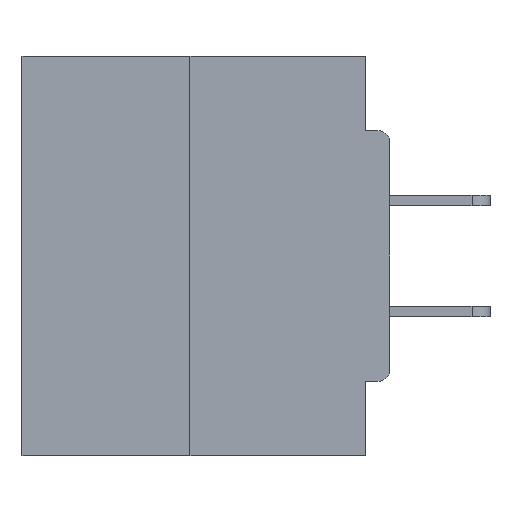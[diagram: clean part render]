
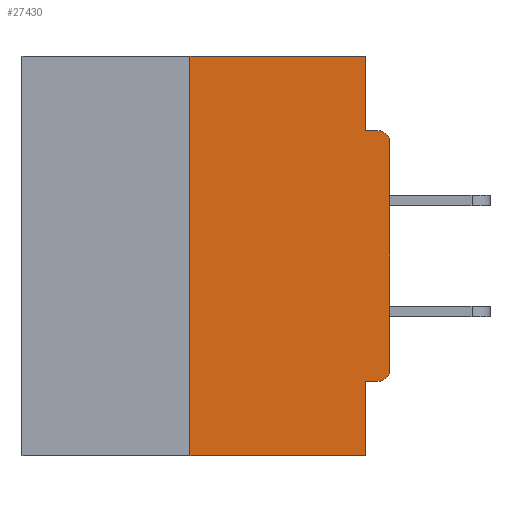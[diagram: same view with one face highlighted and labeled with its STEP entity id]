
A CAD part, left-side view. The second image highlights one B-rep face of the part: STEP entity #27430.
In plain terms, the highlighted planar face has unit normal (-1, 0, 0).
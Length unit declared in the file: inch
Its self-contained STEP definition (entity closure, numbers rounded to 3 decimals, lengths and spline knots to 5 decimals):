
#568 = CARTESIAN_POINT ( 'NONE',  ( 0., 0., -0.4065 ) ) ;
#651 = DIRECTION ( 'NONE',  ( 0., -1., 0. ) ) ;
#1003 = PLANE ( 'NONE',  #7774 ) ;
#1211 = VERTEX_POINT ( 'NONE', #4694 ) ;
#1562 = VERTEX_POINT ( 'NONE', #13886 ) ;
#2189 = CIRCLE ( 'NONE', #25686, 0.015 ) ;
#3286 = VECTOR ( 'NONE', #24534, 39.37008 ) ;
#3760 = VERTEX_POINT ( 'NONE', #14637 ) ;
#3921 = DIRECTION ( 'NONE',  ( 0., 0., -1. ) ) ;
#4142 = EDGE_CURVE ( 'NONE', #23697, #5445, #2189, .T. ) ;
#4460 = CARTESIAN_POINT ( 'NONE',  ( 0., 0.015, -0.1085 ) ) ;
#4552 = LINE ( 'NONE', #12331, #5363 ) ;
#4583 = LINE ( 'NONE', #19253, #12326 ) ;
#4694 = CARTESIAN_POINT ( 'NONE',  ( 0., 0.25, -0.5 ) ) ;
#4850 = DIRECTION ( 'NONE',  ( 0., 0., -1. ) ) ;
#4915 = EDGE_CURVE ( 'NONE', #1211, #28017, #23718, .T. ) ;
#5363 = VECTOR ( 'NONE', #28226, 39.37008 ) ;
#5445 = VERTEX_POINT ( 'NONE', #30517 ) ;
#5545 = EDGE_CURVE ( 'NONE', #1211, #30929, #17136, .T. ) ;
#7144 = LINE ( 'NONE', #28218, #26392 ) ;
#7532 = CIRCLE ( 'NONE', #31305, 0.015 ) ;
#7774 = AXIS2_PLACEMENT_3D ( 'NONE', #29403, #24386, #29758 ) ;
#8301 = VERTEX_POINT ( 'NONE', #27551 ) ;
#8488 = DIRECTION ( 'NONE',  ( 0., 0., -1. ) ) ;
#8930 = CARTESIAN_POINT ( 'NONE',  ( 0., 0.25, 0. ) ) ;
#9136 = CARTESIAN_POINT ( 'NONE',  ( 0., 0.031, -0.5 ) ) ;
#9816 = LINE ( 'NONE', #568, #31940 ) ;
#11010 = DIRECTION ( 'NONE',  ( 0., 1., 0. ) ) ;
#11170 = ORIENTED_EDGE ( 'NONE', *, *, #29361, .T. ) ;
#11292 = EDGE_CURVE ( 'NONE', #30929, #8301, #4552, .T. ) ;
#11531 = ORIENTED_EDGE ( 'NONE', *, *, #11292, .F. ) ;
#11985 = DIRECTION ( 'NONE',  ( -1., 0., 0. ) ) ;
#12326 = VECTOR ( 'NONE', #8488, 39.37008 ) ;
#12327 = VECTOR ( 'NONE', #20142, 39.37008 ) ;
#12331 = CARTESIAN_POINT ( 'NONE',  ( 0., 0.46, 0. ) ) ;
#13746 = CARTESIAN_POINT ( 'NONE',  ( 0., 0.031, -0.0935 ) ) ;
#13886 = CARTESIAN_POINT ( 'NONE',  ( 0., 0.015, -0.4065 ) ) ;
#13926 = CARTESIAN_POINT ( 'NONE',  ( 0., 0., -0.1085 ) ) ;
#13943 = DIRECTION ( 'NONE',  ( -1., 0., 0. ) ) ;
#14561 = ORIENTED_EDGE ( 'NONE', *, *, #5545, .F. ) ;
#14637 = CARTESIAN_POINT ( 'NONE',  ( 0., 0., -0.3915 ) ) ;
#14647 = ORIENTED_EDGE ( 'NONE', *, *, #23054, .F. ) ;
#14877 = CARTESIAN_POINT ( 'NONE',  ( 0., 0., 0. ) ) ;
#15485 = FACE_OUTER_BOUND ( 'NONE', #21297, .T. ) ;
#15745 = DIRECTION ( 'NONE',  ( 0., -1., 0. ) ) ;
#16427 = EDGE_CURVE ( 'NONE', #27950, #5445, #7144, .T. ) ;
#17136 = LINE ( 'NONE', #8930, #3286 ) ;
#18303 = EDGE_CURVE ( 'NONE', #8301, #27950, #4583, .T. ) ;
#19253 = CARTESIAN_POINT ( 'NONE',  ( 0., 0.031, 0. ) ) ;
#19520 = ORIENTED_EDGE ( 'NONE', *, *, #18303, .F. ) ;
#19886 = DIRECTION ( 'NONE',  ( 0., 0., -1. ) ) ;
#19942 = EDGE_CURVE ( 'NONE', #29786, #28017, #23563, .T. ) ;
#20058 = ORIENTED_EDGE ( 'NONE', *, *, #26001, .T. ) ;
#20142 = DIRECTION ( 'NONE',  ( 0., 0., 1. ) ) ;
#21297 = EDGE_LOOP ( 'NONE', ( #11531, #14561, #33757, #28497, #14647, #11170, #20058, #25722, #33706, #19520 ) ) ;
#23054 = EDGE_CURVE ( 'NONE', #1562, #29786, #9816, .T. ) ;
#23563 = LINE ( 'NONE', #30910, #31347 ) ;
#23647 = CARTESIAN_POINT ( 'NONE',  ( 0., 0.031, -0.4065 ) ) ;
#23697 = VERTEX_POINT ( 'NONE', #13926 ) ;
#23718 = LINE ( 'NONE', #28482, #24555 ) ;
#24386 = DIRECTION ( 'NONE',  ( 1., 0., 0. ) ) ;
#24534 = DIRECTION ( 'NONE',  ( 0., 0., 1. ) ) ;
#24555 = VECTOR ( 'NONE', #651, 39.37008 ) ;
#25686 = AXIS2_PLACEMENT_3D ( 'NONE', #4460, #11985, #19886 ) ;
#25722 = ORIENTED_EDGE ( 'NONE', *, *, #4142, .T. ) ;
#26001 = EDGE_CURVE ( 'NONE', #3760, #23697, #29540, .T. ) ;
#26392 = VECTOR ( 'NONE', #15745, 39.37008 ) ;
#27430 = ADVANCED_FACE ( 'NONE', ( #15485 ), #1003, .F. ) ;
#27551 = CARTESIAN_POINT ( 'NONE',  ( 0., 0.031, 0. ) ) ;
#27950 = VERTEX_POINT ( 'NONE', #13746 ) ;
#28017 = VERTEX_POINT ( 'NONE', #9136 ) ;
#28218 = CARTESIAN_POINT ( 'NONE',  ( 0., 0., -0.0935 ) ) ;
#28226 = DIRECTION ( 'NONE',  ( 0., -1., 0. ) ) ;
#28482 = CARTESIAN_POINT ( 'NONE',  ( 0., 0.46, -0.5 ) ) ;
#28497 = ORIENTED_EDGE ( 'NONE', *, *, #19942, .F. ) ;
#29361 = EDGE_CURVE ( 'NONE', #1562, #3760, #7532, .T. ) ;
#29403 = CARTESIAN_POINT ( 'NONE',  ( 0., 0.46, 0. ) ) ;
#29515 = CARTESIAN_POINT ( 'NONE',  ( 0., 0.015, -0.3915 ) ) ;
#29540 = LINE ( 'NONE', #14877, #12327 ) ;
#29758 = DIRECTION ( 'NONE',  ( 0., 0., -1. ) ) ;
#29786 = VERTEX_POINT ( 'NONE', #23647 ) ;
#30517 = CARTESIAN_POINT ( 'NONE',  ( 0., 0.015, -0.0935 ) ) ;
#30910 = CARTESIAN_POINT ( 'NONE',  ( 0., 0.031, -0.5 ) ) ;
#30929 = VERTEX_POINT ( 'NONE', #33640 ) ;
#31305 = AXIS2_PLACEMENT_3D ( 'NONE', #29515, #13943, #3921 ) ;
#31347 = VECTOR ( 'NONE', #4850, 39.37008 ) ;
#31940 = VECTOR ( 'NONE', #11010, 39.37008 ) ;
#33640 = CARTESIAN_POINT ( 'NONE',  ( 0., 0.25, 0. ) ) ;
#33706 = ORIENTED_EDGE ( 'NONE', *, *, #16427, .F. ) ;
#33757 = ORIENTED_EDGE ( 'NONE', *, *, #4915, .T. ) ;
